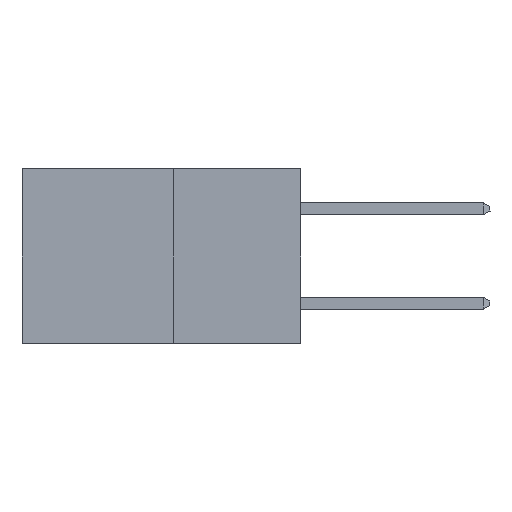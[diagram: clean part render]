
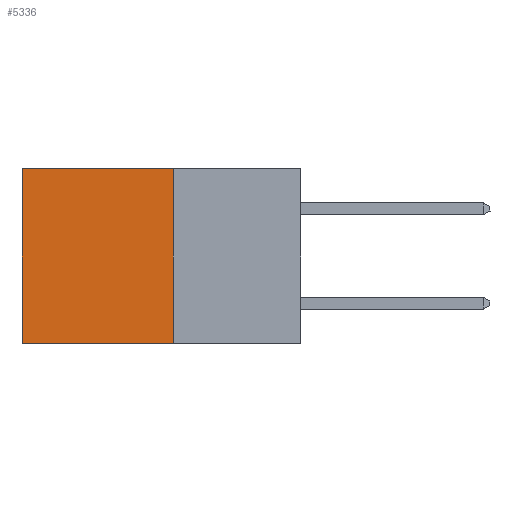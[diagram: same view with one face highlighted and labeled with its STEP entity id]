
A CAD part, left-side view. The second image highlights one B-rep face of the part: STEP entity #5336.
In plain terms, the highlighted planar face has unit normal (-1, 0, 0).
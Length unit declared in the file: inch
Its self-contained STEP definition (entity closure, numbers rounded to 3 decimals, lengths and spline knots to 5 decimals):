
#1130 = ORIENTED_EDGE ( 'NONE', *, *, #21985, .T. ) ;
#2391 = LINE ( 'NONE', #7797, #7227 ) ;
#5101 = VECTOR ( 'NONE', #12655, 39.37008 ) ;
#5336 = ADVANCED_FACE ( 'NONE', ( #12761 ), #17228, .F. ) ;
#5435 = ORIENTED_EDGE ( 'NONE', *, *, #13949, .F. ) ;
#7104 = LINE ( 'NONE', #13589, #17206 ) ;
#7227 = VECTOR ( 'NONE', #9856, 39.37008 ) ;
#7713 = ORIENTED_EDGE ( 'NONE', *, *, #12128, .T. ) ;
#7797 = CARTESIAN_POINT ( 'NONE',  ( 0.277, 0.27, 0. ) ) ;
#7983 = VERTEX_POINT ( 'NONE', #12819 ) ;
#8580 = CARTESIAN_POINT ( 'NONE',  ( 0.277, 0.27, 0. ) ) ;
#9257 = DIRECTION ( 'NONE',  ( 0., 0., -1. ) ) ;
#9856 = DIRECTION ( 'NONE',  ( 0., 1., 0. ) ) ;
#10154 = VERTEX_POINT ( 'NONE', #20370 ) ;
#10698 = CARTESIAN_POINT ( 'NONE',  ( 0.277, 0.27, -0.37 ) ) ;
#11216 = CARTESIAN_POINT ( 'NONE',  ( 0.277, 0.27, -0.37 ) ) ;
#12128 = EDGE_CURVE ( 'NONE', #19321, #18585, #2391, .T. ) ;
#12655 = DIRECTION ( 'NONE',  ( 0., 0., -1. ) ) ;
#12761 = FACE_OUTER_BOUND ( 'NONE', #25292, .T. ) ;
#12819 = CARTESIAN_POINT ( 'NONE',  ( 0.277, 0.59, -0.37 ) ) ;
#13250 = DIRECTION ( 'NONE',  ( 0., 1., 0. ) ) ;
#13589 = CARTESIAN_POINT ( 'NONE',  ( 0.277, 0.59, -0.37 ) ) ;
#13949 = EDGE_CURVE ( 'NONE', #10154, #7983, #17862, .T. ) ;
#15962 = LINE ( 'NONE', #10698, #5101 ) ;
#16694 = AXIS2_PLACEMENT_3D ( 'NONE', #19236, #21177, #9257 ) ;
#17206 = VECTOR ( 'NONE', #17529, 39.37008 ) ;
#17223 = VECTOR ( 'NONE', #13250, 39.37008 ) ;
#17228 = PLANE ( 'NONE',  #16694 ) ;
#17529 = DIRECTION ( 'NONE',  ( 0., 0., -1. ) ) ;
#17862 = LINE ( 'NONE', #11216, #17223 ) ;
#18013 = CARTESIAN_POINT ( 'NONE',  ( 0.277, 0.59, 0. ) ) ;
#18585 = VERTEX_POINT ( 'NONE', #18013 ) ;
#19236 = CARTESIAN_POINT ( 'NONE',  ( 0.277, 0.27, -0.37 ) ) ;
#19321 = VERTEX_POINT ( 'NONE', #8580 ) ;
#20370 = CARTESIAN_POINT ( 'NONE',  ( 0.277, 0.27, -0.37 ) ) ;
#21177 = DIRECTION ( 'NONE',  ( 1., 0., 0. ) ) ;
#21985 = EDGE_CURVE ( 'NONE', #18585, #7983, #7104, .T. ) ;
#23065 = EDGE_CURVE ( 'NONE', #19321, #10154, #15962, .T. ) ;
#25292 = EDGE_LOOP ( 'NONE', ( #1130, #5435, #25765, #7713 ) ) ;
#25765 = ORIENTED_EDGE ( 'NONE', *, *, #23065, .F. ) ;
